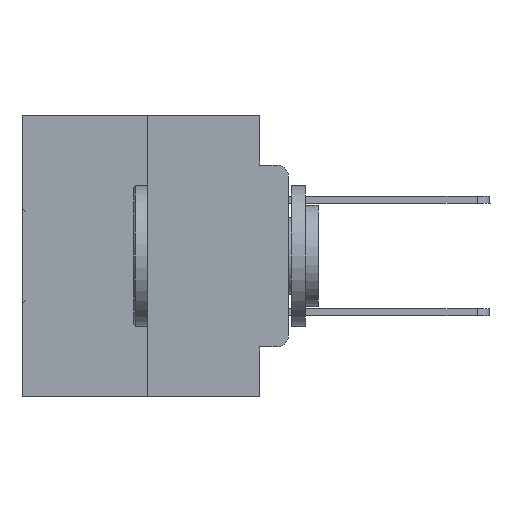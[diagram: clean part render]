
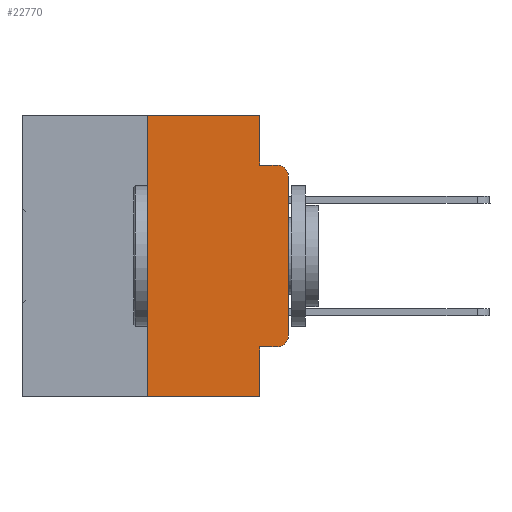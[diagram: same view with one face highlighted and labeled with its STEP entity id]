
A CAD part, left-side view. The second image highlights one B-rep face of the part: STEP entity #22770.
In plain terms, the highlighted planar face has unit normal (-1, 0, 0).
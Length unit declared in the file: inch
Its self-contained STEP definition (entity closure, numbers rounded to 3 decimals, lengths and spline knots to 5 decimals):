
#54 = DIRECTION ( 'NONE',  ( 0., 0., -1. ) ) ;
#487 = EDGE_CURVE ( 'NONE', #24595, #1631, #18597, .T. ) ;
#721 = CARTESIAN_POINT ( 'NONE',  ( 0., 0.25, 0. ) ) ;
#976 = CARTESIAN_POINT ( 'NONE',  ( 0., 0.02, -0.4115 ) ) ;
#1631 = VERTEX_POINT ( 'NONE', #6294 ) ;
#2068 = DIRECTION ( 'NONE',  ( 0., -1., 0. ) ) ;
#2372 = VERTEX_POINT ( 'NONE', #22568 ) ;
#3686 = VERTEX_POINT ( 'NONE', #19939 ) ;
#3963 = VERTEX_POINT ( 'NONE', #13356 ) ;
#4523 = ORIENTED_EDGE ( 'NONE', *, *, #28901, .F. ) ;
#4582 = CARTESIAN_POINT ( 'NONE',  ( 0., 0.473, -0.5 ) ) ;
#4813 = DIRECTION ( 'NONE',  ( 0., 0., -1. ) ) ;
#5305 = ORIENTED_EDGE ( 'NONE', *, *, #487, .T. ) ;
#5737 = EDGE_CURVE ( 'NONE', #10481, #24595, #24393, .T. ) ;
#6294 = CARTESIAN_POINT ( 'NONE',  ( 0., 0.02, -0.0885 ) ) ;
#7231 = CARTESIAN_POINT ( 'NONE',  ( 0., 0., -0.3915 ) ) ;
#7469 = LINE ( 'NONE', #25777, #13591 ) ;
#7617 = DIRECTION ( 'NONE',  ( 0., 0., 1. ) ) ;
#8561 = CARTESIAN_POINT ( 'NONE',  ( 0., 0.25, 0. ) ) ;
#8825 = FACE_OUTER_BOUND ( 'NONE', #14713, .T. ) ;
#9319 = ORIENTED_EDGE ( 'NONE', *, *, #9849, .T. ) ;
#9585 = VECTOR ( 'NONE', #28482, 39.37008 ) ;
#9816 = VECTOR ( 'NONE', #7617, 39.37008 ) ;
#9849 = EDGE_CURVE ( 'NONE', #11808, #10481, #20566, .T. ) ;
#9875 = CARTESIAN_POINT ( 'NONE',  ( 0., 0.051, -0.0885 ) ) ;
#10102 = CARTESIAN_POINT ( 'NONE',  ( 0., 0.02, -0.3915 ) ) ;
#10245 = LINE ( 'NONE', #8561, #16359 ) ;
#10457 = PLANE ( 'NONE',  #27770 ) ;
#10464 = CARTESIAN_POINT ( 'NONE',  ( 0., 0., -0.1085 ) ) ;
#10481 = VERTEX_POINT ( 'NONE', #7231 ) ;
#10719 = VECTOR ( 'NONE', #22794, 39.37008 ) ;
#11432 = EDGE_CURVE ( 'NONE', #16949, #25035, #20931, .T. ) ;
#11488 = VECTOR ( 'NONE', #27233, 39.37008 ) ;
#11543 = AXIS2_PLACEMENT_3D ( 'NONE', #14682, #14695, #4813 ) ;
#11808 = VERTEX_POINT ( 'NONE', #976 ) ;
#11947 = CARTESIAN_POINT ( 'NONE',  ( 0., 0.051, 0. ) ) ;
#12397 = CARTESIAN_POINT ( 'NONE',  ( 0., 0.051, -0.5 ) ) ;
#12537 = CARTESIAN_POINT ( 'NONE',  ( 0., 0.473, 0. ) ) ;
#12773 = DIRECTION ( 'NONE',  ( 0., 0., -1. ) ) ;
#13098 = CARTESIAN_POINT ( 'NONE',  ( 0., 0.051, -0.4115 ) ) ;
#13105 = CARTESIAN_POINT ( 'NONE',  ( 0., 0.473, 0. ) ) ;
#13356 = CARTESIAN_POINT ( 'NONE',  ( 0., 0.051, -0.0885 ) ) ;
#13591 = VECTOR ( 'NONE', #15581, 39.37008 ) ;
#14076 = VECTOR ( 'NONE', #2068, 39.37008 ) ;
#14682 = CARTESIAN_POINT ( 'NONE',  ( 0., 0.02, -0.1085 ) ) ;
#14695 = DIRECTION ( 'NONE',  ( -1., 0., 0. ) ) ;
#14713 = EDGE_LOOP ( 'NONE', ( #29917, #5305, #25104, #4523, #24313, #30291, #22716, #27089, #17081, #9319 ) ) ;
#14722 = EDGE_CURVE ( 'NONE', #23608, #3686, #18762, .T. ) ;
#15581 = DIRECTION ( 'NONE',  ( 0., 0., -1. ) ) ;
#15700 = DIRECTION ( 'NONE',  ( 1., 0., 0. ) ) ;
#16359 = VECTOR ( 'NONE', #24064, 39.37008 ) ;
#16531 = LINE ( 'NONE', #13098, #9585 ) ;
#16846 = EDGE_CURVE ( 'NONE', #2372, #11808, #16531, .T. ) ;
#16949 = VERTEX_POINT ( 'NONE', #26328 ) ;
#16973 = AXIS2_PLACEMENT_3D ( 'NONE', #10102, #28144, #12773 ) ;
#17081 = ORIENTED_EDGE ( 'NONE', *, *, #16846, .T. ) ;
#18597 = CIRCLE ( 'NONE', #11543, 0.02 ) ;
#18612 = EDGE_CURVE ( 'NONE', #2372, #25035, #7469, .T. ) ;
#18762 = LINE ( 'NONE', #12537, #31482 ) ;
#19939 = CARTESIAN_POINT ( 'NONE',  ( 0., 0.051, 0. ) ) ;
#20326 = EDGE_CURVE ( 'NONE', #16949, #23608, #10245, .T. ) ;
#20566 = CIRCLE ( 'NONE', #16973, 0.02 ) ;
#20931 = LINE ( 'NONE', #4582, #14076 ) ;
#22568 = CARTESIAN_POINT ( 'NONE',  ( 0., 0.051, -0.4115 ) ) ;
#22716 = ORIENTED_EDGE ( 'NONE', *, *, #11432, .T. ) ;
#22770 = ADVANCED_FACE ( 'NONE', ( #8825 ), #10457, .F. ) ;
#22772 = DIRECTION ( 'NONE',  ( 0., -1., 0. ) ) ;
#22794 = DIRECTION ( 'NONE',  ( 0., -1., 0. ) ) ;
#23608 = VERTEX_POINT ( 'NONE', #721 ) ;
#24064 = DIRECTION ( 'NONE',  ( 0., 0., 1. ) ) ;
#24313 = ORIENTED_EDGE ( 'NONE', *, *, #14722, .F. ) ;
#24393 = LINE ( 'NONE', #25678, #9816 ) ;
#24595 = VERTEX_POINT ( 'NONE', #10464 ) ;
#25035 = VERTEX_POINT ( 'NONE', #12397 ) ;
#25104 = ORIENTED_EDGE ( 'NONE', *, *, #32218, .F. ) ;
#25196 = LINE ( 'NONE', #11947, #11488 ) ;
#25678 = CARTESIAN_POINT ( 'NONE',  ( 0., 0., 0. ) ) ;
#25777 = CARTESIAN_POINT ( 'NONE',  ( 0., 0.051, 0. ) ) ;
#26328 = CARTESIAN_POINT ( 'NONE',  ( 0., 0.25, -0.5 ) ) ;
#27089 = ORIENTED_EDGE ( 'NONE', *, *, #18612, .F. ) ;
#27233 = DIRECTION ( 'NONE',  ( 0., 0., -1. ) ) ;
#27770 = AXIS2_PLACEMENT_3D ( 'NONE', #13105, #15700, #54 ) ;
#28144 = DIRECTION ( 'NONE',  ( -1., 0., 0. ) ) ;
#28482 = DIRECTION ( 'NONE',  ( 0., -1., 0. ) ) ;
#28901 = EDGE_CURVE ( 'NONE', #3686, #3963, #25196, .T. ) ;
#29917 = ORIENTED_EDGE ( 'NONE', *, *, #5737, .T. ) ;
#30291 = ORIENTED_EDGE ( 'NONE', *, *, #20326, .F. ) ;
#31482 = VECTOR ( 'NONE', #22772, 39.37008 ) ;
#31962 = LINE ( 'NONE', #9875, #10719 ) ;
#32218 = EDGE_CURVE ( 'NONE', #3963, #1631, #31962, .T. ) ;
